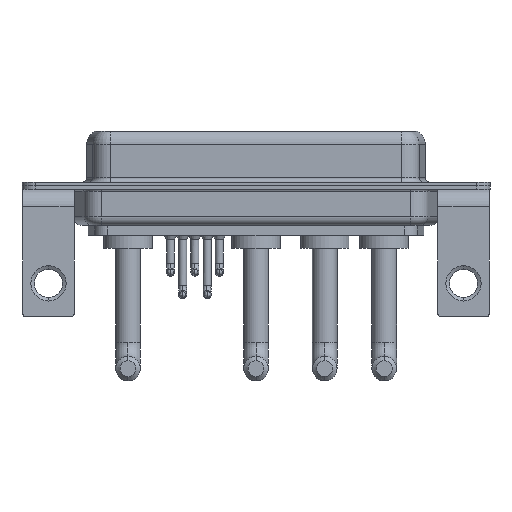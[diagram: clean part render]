
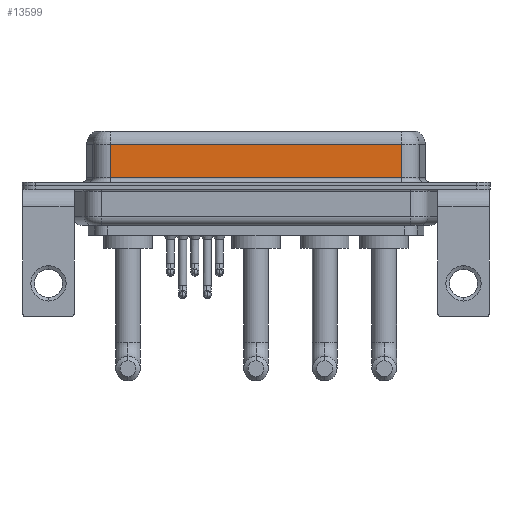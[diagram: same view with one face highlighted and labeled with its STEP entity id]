
A CAD part, front view. The second image highlights one B-rep face of the part: STEP entity #13599.
In plain terms, the highlighted planar face has unit normal (0, -1, 0).
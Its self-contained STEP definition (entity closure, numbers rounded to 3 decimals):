
#977 = CARTESIAN_POINT ( 'NONE',  ( 7.013, -3.95, 6.4 ) ) ;
#2212 = VERTEX_POINT ( 'NONE', #5996 ) ;
#2471 = LINE ( 'NONE', #10511, #12676 ) ;
#3135 = ORIENTED_EDGE ( 'NONE', *, *, #8914, .T. ) ;
#3429 = LINE ( 'NONE', #9004, #13778 ) ;
#3801 = DIRECTION ( 'NONE',  ( 0., 0., -1. ) ) ;
#4061 = CARTESIAN_POINT ( 'NONE',  ( 40.037, -3.95, 0.9 ) ) ;
#4145 = LINE ( 'NONE', #4061, #8630 ) ;
#4412 = CARTESIAN_POINT ( 'NONE',  ( 40.037, -3.95, 4.65 ) ) ;
#5127 = EDGE_CURVE ( 'NONE', #17689, #2212, #4145, .T. ) ;
#5345 = DIRECTION ( 'NONE',  ( 1., 0., 0. ) ) ;
#5495 = CARTESIAN_POINT ( 'NONE',  ( 40.037, -3.95, 6.4 ) ) ;
#5996 = CARTESIAN_POINT ( 'NONE',  ( 40.037, -3.95, 0.9 ) ) ;
#6163 = DIRECTION ( 'NONE',  ( -1., 0., 0. ) ) ;
#7901 = LINE ( 'NONE', #977, #15499 ) ;
#7963 = VERTEX_POINT ( 'NONE', #13318 ) ;
#8240 = EDGE_CURVE ( 'NONE', #7963, #17689, #7901, .T. ) ;
#8630 = VECTOR ( 'NONE', #5345, 1000. ) ;
#8914 = EDGE_CURVE ( 'NONE', #14083, #7963, #3429, .T. ) ;
#9004 = CARTESIAN_POINT ( 'NONE',  ( 40.037, -3.95, 4.65 ) ) ;
#9172 = ORIENTED_EDGE ( 'NONE', *, *, #5127, .T. ) ;
#10035 = DIRECTION ( 'NONE',  ( 0., 0., 1. ) ) ;
#10511 = CARTESIAN_POINT ( 'NONE',  ( 40.037, -3.95, 6.4 ) ) ;
#10613 = EDGE_LOOP ( 'NONE', ( #15271, #3135, #13077, #9172 ) ) ;
#11872 = EDGE_CURVE ( 'NONE', #14083, #2212, #2471, .T. ) ;
#12428 = FACE_OUTER_BOUND ( 'NONE', #10613, .T. ) ;
#12676 = VECTOR ( 'NONE', #13572, 1000. ) ;
#13077 = ORIENTED_EDGE ( 'NONE', *, *, #8240, .T. ) ;
#13318 = CARTESIAN_POINT ( 'NONE',  ( 7.013, -3.95, 4.65 ) ) ;
#13572 = DIRECTION ( 'NONE',  ( 0., 0., -1. ) ) ;
#13599 = ADVANCED_FACE ( 'NONE', ( #12428 ), #14961, .F. ) ;
#13778 = VECTOR ( 'NONE', #6163, 1000. ) ;
#14083 = VERTEX_POINT ( 'NONE', #4412 ) ;
#14190 = DIRECTION ( 'NONE',  ( 0., 1., 0. ) ) ;
#14206 = CARTESIAN_POINT ( 'NONE',  ( 7.013, -3.95, 0.9 ) ) ;
#14961 = PLANE ( 'NONE',  #15608 ) ;
#15271 = ORIENTED_EDGE ( 'NONE', *, *, #11872, .F. ) ;
#15499 = VECTOR ( 'NONE', #3801, 1000. ) ;
#15608 = AXIS2_PLACEMENT_3D ( 'NONE', #5495, #14190, #10035 ) ;
#17689 = VERTEX_POINT ( 'NONE', #14206 ) ;
